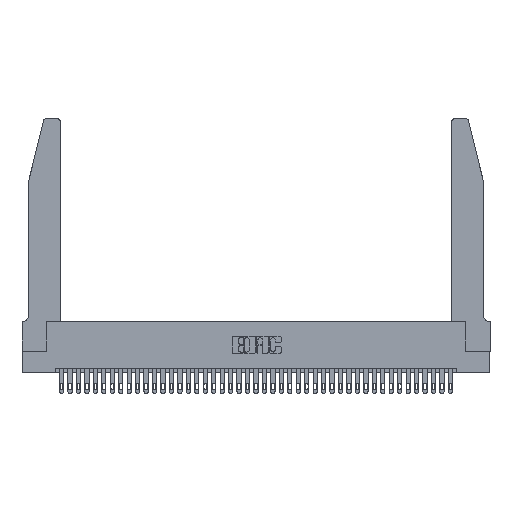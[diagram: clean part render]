
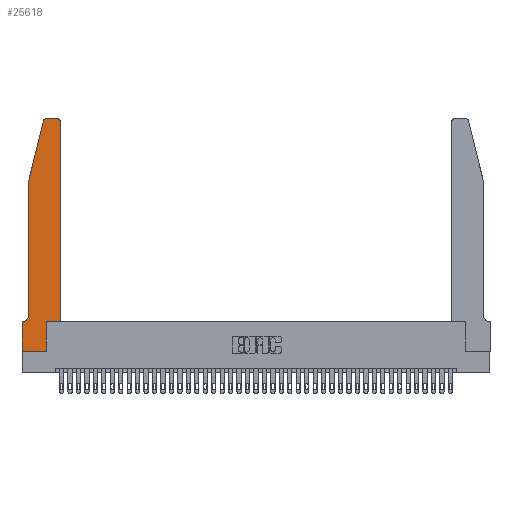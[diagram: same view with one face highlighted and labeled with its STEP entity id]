
A CAD part, top view. The second image highlights one B-rep face of the part: STEP entity #25618.
In plain terms, the highlighted planar face has unit normal (0, 0, 1).
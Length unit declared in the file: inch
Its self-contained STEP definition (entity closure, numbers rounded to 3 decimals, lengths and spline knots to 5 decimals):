
#147 = VECTOR ( 'NONE', #11840, 39.37008 ) ;
#597 = CARTESIAN_POINT ( 'NONE',  ( 0., 0., 0.37 ) ) ;
#1024 = CIRCLE ( 'NONE', #20411, 0.03 ) ;
#1073 = VERTEX_POINT ( 'NONE', #39107 ) ;
#1396 = CARTESIAN_POINT ( 'NONE',  ( 0.4505, 0.35, 0.37 ) ) ;
#1739 = CARTESIAN_POINT ( 'NONE',  ( 0., 0.35, 0.37 ) ) ;
#2052 = EDGE_CURVE ( 'NONE', #12076, #33010, #17766, .T. ) ;
#2375 = ORIENTED_EDGE ( 'NONE', *, *, #2052, .T. ) ;
#2503 = CARTESIAN_POINT ( 'NONE',  ( 0., 0., 0.37 ) ) ;
#2746 = CARTESIAN_POINT ( 'NONE',  ( 0., 0.35, 0.37 ) ) ;
#3165 = VECTOR ( 'NONE', #15818, 39.37008 ) ;
#3482 = EDGE_CURVE ( 'NONE', #1073, #12076, #31441, .T. ) ;
#4109 = CARTESIAN_POINT ( 'NONE',  ( 0.0755, 2., 0.37 ) ) ;
#4137 = EDGE_CURVE ( 'NONE', #19134, #1073, #22932, .T. ) ;
#5679 = EDGE_CURVE ( 'NONE', #6888, #18299, #15222, .T. ) ;
#5900 = DIRECTION ( 'NONE',  ( -0.239, -0.971, 0. ) ) ;
#6094 = DIRECTION ( 'NONE',  ( 0., 0., -1. ) ) ;
#6888 = VERTEX_POINT ( 'NONE', #15051 ) ;
#7791 = DIRECTION ( 'NONE',  ( 1., 0., 0. ) ) ;
#8008 = LINE ( 'NONE', #24852, #15456 ) ;
#9239 = CARTESIAN_POINT ( 'NONE',  ( 0.4505, 0.35, 0.37 ) ) ;
#9602 = ORIENTED_EDGE ( 'NONE', *, *, #5679, .T. ) ;
#10607 = ORIENTED_EDGE ( 'NONE', *, *, #21629, .T. ) ;
#10794 = VECTOR ( 'NONE', #16614, 39.37008 ) ;
#10799 = CARTESIAN_POINT ( 'NONE',  ( 0.25487, 2.72718, 0.37 ) ) ;
#10964 = AXIS2_PLACEMENT_3D ( 'NONE', #32370, #35301, #38453 ) ;
#11684 = EDGE_CURVE ( 'NONE', #26185, #30070, #8008, .T. ) ;
#11840 = DIRECTION ( 'NONE',  ( 0., 1., 0. ) ) ;
#12076 = VERTEX_POINT ( 'NONE', #9239 ) ;
#12677 = EDGE_CURVE ( 'NONE', #33010, #6888, #14083, .T. ) ;
#13504 = AXIS2_PLACEMENT_3D ( 'NONE', #1739, #29590, #7791 ) ;
#13564 = EDGE_CURVE ( 'NONE', #17997, #40818, #36274, .T. ) ;
#13714 = LINE ( 'NONE', #4109, #20704 ) ;
#14083 = CIRCLE ( 'NONE', #10964, 0.03 ) ;
#15046 = CARTESIAN_POINT ( 'NONE',  ( 0.2865, 0., 0.37 ) ) ;
#15051 = CARTESIAN_POINT ( 'NONE',  ( 0.4205, 2.75, 0.37 ) ) ;
#15222 = LINE ( 'NONE', #30798, #21161 ) ;
#15456 = VECTOR ( 'NONE', #5900, 39.37008 ) ;
#15818 = DIRECTION ( 'NONE',  ( -1., 0., 0. ) ) ;
#16614 = DIRECTION ( 'NONE',  ( 0., 1., 0. ) ) ;
#16630 = VECTOR ( 'NONE', #28292, 39.37008 ) ;
#17310 = DIRECTION ( 'NONE',  ( 1., 0., 0. ) ) ;
#17766 = LINE ( 'NONE', #1396, #10794 ) ;
#17997 = VERTEX_POINT ( 'NONE', #24698 ) ;
#18151 = DIRECTION ( 'NONE',  ( -1., 0., 0. ) ) ;
#18299 = VERTEX_POINT ( 'NONE', #37358 ) ;
#19111 = EDGE_CURVE ( 'NONE', #32487, #19134, #34991, .T. ) ;
#19134 = VERTEX_POINT ( 'NONE', #15046 ) ;
#19859 = VERTEX_POINT ( 'NONE', #2746 ) ;
#20243 = DIRECTION ( 'NONE',  ( 0., 0., 1. ) ) ;
#20411 = AXIS2_PLACEMENT_3D ( 'NONE', #29545, #20243, #17310 ) ;
#20468 = LINE ( 'NONE', #35849, #3165 ) ;
#20704 = VECTOR ( 'NONE', #29339, 39.37008 ) ;
#21161 = VECTOR ( 'NONE', #18151, 39.37008 ) ;
#21584 = DIRECTION ( 'NONE',  ( 1., 0., 0. ) ) ;
#21629 = EDGE_CURVE ( 'NONE', #40818, #19859, #20468, .T. ) ;
#21903 = ORIENTED_EDGE ( 'NONE', *, *, #4137, .T. ) ;
#22400 = EDGE_CURVE ( 'NONE', #19859, #32487, #36235, .T. ) ;
#22592 = ORIENTED_EDGE ( 'NONE', *, *, #23062, .T. ) ;
#22674 = CARTESIAN_POINT ( 'NONE',  ( 0.4505, 2.72, 0.37 ) ) ;
#22932 = LINE ( 'NONE', #30706, #147 ) ;
#22955 = ORIENTED_EDGE ( 'NONE', *, *, #22400, .T. ) ;
#23062 = EDGE_CURVE ( 'NONE', #18299, #26185, #1024, .T. ) ;
#24380 = FACE_OUTER_BOUND ( 'NONE', #37952, .T. ) ;
#24698 = CARTESIAN_POINT ( 'NONE',  ( 0.0755, 0.42, 0.37 ) ) ;
#24852 = CARTESIAN_POINT ( 'NONE',  ( 0.0755, 2., 0.37 ) ) ;
#25067 = EDGE_CURVE ( 'NONE', #30070, #17997, #13714, .T. ) ;
#25395 = CARTESIAN_POINT ( 'NONE',  ( 0.4505, 0.35, 0.37 ) ) ;
#25618 = ADVANCED_FACE ( 'NONE', ( #24380 ), #36435, .T. ) ;
#25917 = DIRECTION ( 'NONE',  ( 0., -1., 0. ) ) ;
#26185 = VERTEX_POINT ( 'NONE', #10799 ) ;
#28189 = DIRECTION ( 'NONE',  ( -1., 0., 0. ) ) ;
#28292 = DIRECTION ( 'NONE',  ( 1., 0., 0. ) ) ;
#28438 = AXIS2_PLACEMENT_3D ( 'NONE', #40492, #6094, #28189 ) ;
#28751 = ORIENTED_EDGE ( 'NONE', *, *, #3482, .T. ) ;
#29339 = DIRECTION ( 'NONE',  ( 0., -1., 0. ) ) ;
#29527 = CARTESIAN_POINT ( 'NONE',  ( 0., 0., 0.37 ) ) ;
#29545 = CARTESIAN_POINT ( 'NONE',  ( 0.284, 2.72, 0.37 ) ) ;
#29590 = DIRECTION ( 'NONE',  ( 0., 0., 1. ) ) ;
#30070 = VERTEX_POINT ( 'NONE', #37424 ) ;
#30706 = CARTESIAN_POINT ( 'NONE',  ( 0.2865, 0.35, 0.37 ) ) ;
#30798 = CARTESIAN_POINT ( 'NONE',  ( 0.2605, 2.75, 0.37 ) ) ;
#31441 = LINE ( 'NONE', #25395, #16630 ) ;
#32370 = CARTESIAN_POINT ( 'NONE',  ( 0.4205, 2.72, 0.37 ) ) ;
#32487 = VERTEX_POINT ( 'NONE', #29527 ) ;
#32495 = VECTOR ( 'NONE', #21584, 39.37008 ) ;
#32851 = ORIENTED_EDGE ( 'NONE', *, *, #25067, .T. ) ;
#32884 = ORIENTED_EDGE ( 'NONE', *, *, #13564, .T. ) ;
#33010 = VERTEX_POINT ( 'NONE', #22674 ) ;
#34741 = VECTOR ( 'NONE', #25917, 39.37008 ) ;
#34991 = LINE ( 'NONE', #2503, #32495 ) ;
#35301 = DIRECTION ( 'NONE',  ( 0., 0., 1. ) ) ;
#35743 = ORIENTED_EDGE ( 'NONE', *, *, #19111, .T. ) ;
#35771 = ORIENTED_EDGE ( 'NONE', *, *, #11684, .T. ) ;
#35849 = CARTESIAN_POINT ( 'NONE',  ( 0.0755, 0.35, 0.37 ) ) ;
#36235 = LINE ( 'NONE', #597, #34741 ) ;
#36274 = CIRCLE ( 'NONE', #28438, 0.07 ) ;
#36435 = PLANE ( 'NONE',  #13504 ) ;
#37358 = CARTESIAN_POINT ( 'NONE',  ( 0.284, 2.75, 0.37 ) ) ;
#37424 = CARTESIAN_POINT ( 'NONE',  ( 0.0755, 2., 0.37 ) ) ;
#37952 = EDGE_LOOP ( 'NONE', ( #9602, #22592, #35771, #32851, #32884, #10607, #22955, #35743, #21903, #28751, #2375, #38296 ) ) ;
#38296 = ORIENTED_EDGE ( 'NONE', *, *, #12677, .T. ) ;
#38453 = DIRECTION ( 'NONE',  ( 1., 0., 0. ) ) ;
#39107 = CARTESIAN_POINT ( 'NONE',  ( 0.2865, 0.35, 0.37 ) ) ;
#39850 = CARTESIAN_POINT ( 'NONE',  ( 0.0055, 0.35, 0.37 ) ) ;
#40492 = CARTESIAN_POINT ( 'NONE',  ( 0.0055, 0.42, 0.37 ) ) ;
#40818 = VERTEX_POINT ( 'NONE', #39850 ) ;
